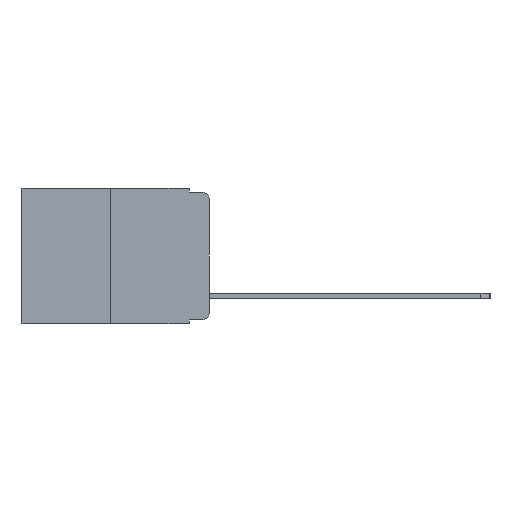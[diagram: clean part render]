
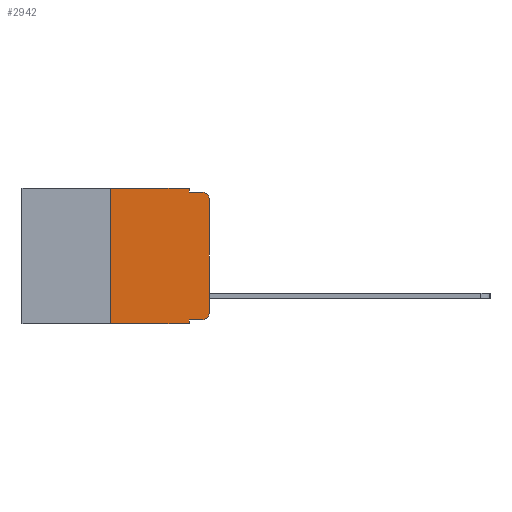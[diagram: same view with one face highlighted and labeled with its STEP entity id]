
A CAD part, left-side view. The second image highlights one B-rep face of the part: STEP entity #2942.
In plain terms, the highlighted planar face has unit normal (-1, 0, 0).
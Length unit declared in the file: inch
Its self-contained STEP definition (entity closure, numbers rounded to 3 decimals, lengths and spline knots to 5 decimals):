
#179 = CARTESIAN_POINT ( 'NONE',  ( 0., 0.02, -0.313 ) ) ;
#488 = CARTESIAN_POINT ( 'NONE',  ( 0., 0., -0.03 ) ) ;
#847 = DIRECTION ( 'NONE',  ( 0., 0., -1. ) ) ;
#909 = LINE ( 'NONE', #8523, #13660 ) ;
#977 = CARTESIAN_POINT ( 'NONE',  ( 0., 0.02, -0.333 ) ) ;
#1303 = DIRECTION ( 'NONE',  ( 0., 0., -1. ) ) ;
#1343 = ORIENTED_EDGE ( 'NONE', *, *, #6800, .T. ) ;
#1538 = VERTEX_POINT ( 'NONE', #2266 ) ;
#1943 = CARTESIAN_POINT ( 'NONE',  ( 0., 0.25, -0.343 ) ) ;
#1955 = CARTESIAN_POINT ( 'NONE',  ( 0., 0.051, 0. ) ) ;
#1985 = ORIENTED_EDGE ( 'NONE', *, *, #11142, .F. ) ;
#2025 = AXIS2_PLACEMENT_3D ( 'NONE', #179, #7837, #1303 ) ;
#2266 = CARTESIAN_POINT ( 'NONE',  ( 0., 0.051, 0. ) ) ;
#2473 = ORIENTED_EDGE ( 'NONE', *, *, #5059, .F. ) ;
#2867 = VECTOR ( 'NONE', #8173, 39.37008 ) ;
#2942 = ADVANCED_FACE ( 'NONE', ( #12955 ), #6242, .F. ) ;
#3073 = AXIS2_PLACEMENT_3D ( 'NONE', #8037, #5404, #7850 ) ;
#3274 = DIRECTION ( 'NONE',  ( 0., 0., -1. ) ) ;
#3473 = LINE ( 'NONE', #6458, #11581 ) ;
#3581 = EDGE_CURVE ( 'NONE', #6087, #7025, #5785, .T. ) ;
#3647 = VERTEX_POINT ( 'NONE', #977 ) ;
#3680 = CARTESIAN_POINT ( 'NONE',  ( 0., 0., -0.313 ) ) ;
#4267 = VERTEX_POINT ( 'NONE', #11504 ) ;
#4379 = CIRCLE ( 'NONE', #2025, 0.02 ) ;
#4982 = AXIS2_PLACEMENT_3D ( 'NONE', #11711, #5445, #12736 ) ;
#5059 = EDGE_CURVE ( 'NONE', #1538, #12644, #10338, .T. ) ;
#5388 = DIRECTION ( 'NONE',  ( 0., -1., 0. ) ) ;
#5404 = DIRECTION ( 'NONE',  ( 1., 0., 0. ) ) ;
#5445 = DIRECTION ( 'NONE',  ( -1., 0., 0. ) ) ;
#5565 = EDGE_CURVE ( 'NONE', #5912, #12507, #13061, .T. ) ;
#5650 = VECTOR ( 'NONE', #5388, 39.37008 ) ;
#5785 = LINE ( 'NONE', #9614, #2867 ) ;
#5912 = VERTEX_POINT ( 'NONE', #13273 ) ;
#6014 = VECTOR ( 'NONE', #8654, 39.37008 ) ;
#6087 = VERTEX_POINT ( 'NONE', #1943 ) ;
#6242 = PLANE ( 'NONE',  #3073 ) ;
#6401 = CIRCLE ( 'NONE', #4982, 0.02 ) ;
#6458 = CARTESIAN_POINT ( 'NONE',  ( 0., 0.473, -0.343 ) ) ;
#6464 = ORIENTED_EDGE ( 'NONE', *, *, #5565, .F. ) ;
#6500 = CARTESIAN_POINT ( 'NONE',  ( 0., 0.473, 0. ) ) ;
#6800 = EDGE_CURVE ( 'NONE', #12457, #7796, #909, .T. ) ;
#6999 = EDGE_CURVE ( 'NONE', #3647, #12457, #4379, .T. ) ;
#7025 = VERTEX_POINT ( 'NONE', #11943 ) ;
#7285 = VECTOR ( 'NONE', #3274, 39.37008 ) ;
#7528 = CARTESIAN_POINT ( 'NONE',  ( 0., 0.051, -0.01 ) ) ;
#7685 = CARTESIAN_POINT ( 'NONE',  ( 0., 0.051, 0. ) ) ;
#7796 = VERTEX_POINT ( 'NONE', #488 ) ;
#7837 = DIRECTION ( 'NONE',  ( -1., 0., 0. ) ) ;
#7850 = DIRECTION ( 'NONE',  ( 0., 0., -1. ) ) ;
#8015 = ORIENTED_EDGE ( 'NONE', *, *, #13126, .F. ) ;
#8036 = ORIENTED_EDGE ( 'NONE', *, *, #11564, .T. ) ;
#8037 = CARTESIAN_POINT ( 'NONE',  ( 0., 0.473, 0. ) ) ;
#8173 = DIRECTION ( 'NONE',  ( 0., 0., 1. ) ) ;
#8523 = CARTESIAN_POINT ( 'NONE',  ( 0., 0., 0. ) ) ;
#8530 = LINE ( 'NONE', #10629, #5650 ) ;
#8654 = DIRECTION ( 'NONE',  ( 0., -1., 0. ) ) ;
#9051 = VECTOR ( 'NONE', #13392, 39.37008 ) ;
#9156 = LINE ( 'NONE', #6500, #6014 ) ;
#9263 = CARTESIAN_POINT ( 'NONE',  ( 0., 0.051, -0.01 ) ) ;
#9524 = DIRECTION ( 'NONE',  ( 0., 0., 1. ) ) ;
#9569 = ORIENTED_EDGE ( 'NONE', *, *, #13304, .T. ) ;
#9609 = DIRECTION ( 'NONE',  ( 0., -1., 0. ) ) ;
#9614 = CARTESIAN_POINT ( 'NONE',  ( 0., 0.25, 0. ) ) ;
#9668 = ORIENTED_EDGE ( 'NONE', *, *, #3581, .F. ) ;
#10289 = EDGE_LOOP ( 'NONE', ( #1343, #11197, #8015, #2473, #1985, #9668, #9569, #6464, #8036, #11037 ) ) ;
#10327 = VECTOR ( 'NONE', #847, 39.37008 ) ;
#10338 = LINE ( 'NONE', #7685, #7285 ) ;
#10629 = CARTESIAN_POINT ( 'NONE',  ( 0., 0.051, -0.333 ) ) ;
#11037 = ORIENTED_EDGE ( 'NONE', *, *, #6999, .T. ) ;
#11142 = EDGE_CURVE ( 'NONE', #7025, #1538, #9156, .T. ) ;
#11197 = ORIENTED_EDGE ( 'NONE', *, *, #13326, .T. ) ;
#11504 = CARTESIAN_POINT ( 'NONE',  ( 0., 0.02, -0.01 ) ) ;
#11564 = EDGE_CURVE ( 'NONE', #5912, #3647, #8530, .T. ) ;
#11581 = VECTOR ( 'NONE', #9609, 39.37008 ) ;
#11711 = CARTESIAN_POINT ( 'NONE',  ( 0., 0.02, -0.03 ) ) ;
#11943 = CARTESIAN_POINT ( 'NONE',  ( 0., 0.25, 0. ) ) ;
#12087 = LINE ( 'NONE', #9263, #9051 ) ;
#12457 = VERTEX_POINT ( 'NONE', #3680 ) ;
#12507 = VERTEX_POINT ( 'NONE', #13267 ) ;
#12644 = VERTEX_POINT ( 'NONE', #7528 ) ;
#12736 = DIRECTION ( 'NONE',  ( 0., 0., -1. ) ) ;
#12955 = FACE_OUTER_BOUND ( 'NONE', #10289, .T. ) ;
#13061 = LINE ( 'NONE', #1955, #10327 ) ;
#13126 = EDGE_CURVE ( 'NONE', #12644, #4267, #12087, .T. ) ;
#13267 = CARTESIAN_POINT ( 'NONE',  ( 0., 0.051, -0.343 ) ) ;
#13273 = CARTESIAN_POINT ( 'NONE',  ( 0., 0.051, -0.333 ) ) ;
#13304 = EDGE_CURVE ( 'NONE', #6087, #12507, #3473, .T. ) ;
#13326 = EDGE_CURVE ( 'NONE', #7796, #4267, #6401, .T. ) ;
#13392 = DIRECTION ( 'NONE',  ( 0., -1., 0. ) ) ;
#13660 = VECTOR ( 'NONE', #9524, 39.37008 ) ;
